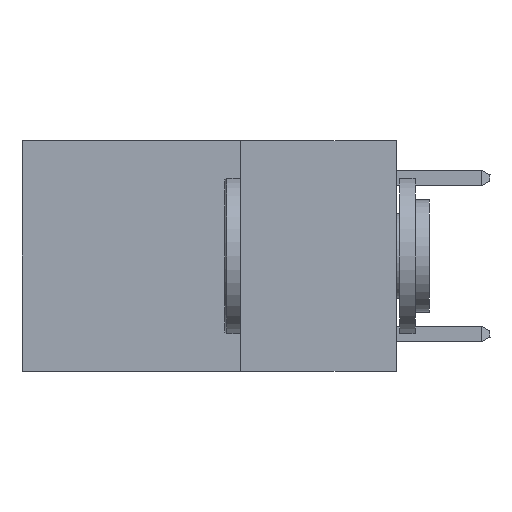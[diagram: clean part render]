
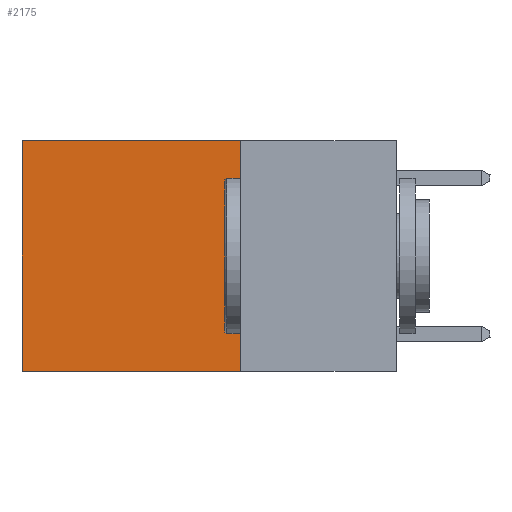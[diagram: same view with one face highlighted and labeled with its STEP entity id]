
A CAD part, left-side view. The second image highlights one B-rep face of the part: STEP entity #2175.
In plain terms, the highlighted planar face has unit normal (-1, 0, 0).
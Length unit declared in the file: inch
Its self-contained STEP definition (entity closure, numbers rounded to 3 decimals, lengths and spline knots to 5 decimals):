
#530 = CARTESIAN_POINT ( 'NONE',  ( 0.2625, 0.25, 0. ) ) ;
#537 = CARTESIAN_POINT ( 'NONE',  ( 0.2625, 0.6, -0.37 ) ) ;
#860 = VERTEX_POINT ( 'NONE', #9631 ) ;
#2175 = ADVANCED_FACE ( 'NONE', ( #6947 ), #11104, .F. ) ;
#2931 = DIRECTION ( 'NONE',  ( 0., 1., 0. ) ) ;
#3820 = ORIENTED_EDGE ( 'NONE', *, *, #22579, .F. ) ;
#5624 = VERTEX_POINT ( 'NONE', #16555 ) ;
#6626 = AXIS2_PLACEMENT_3D ( 'NONE', #17015, #23291, #23563 ) ;
#6947 = FACE_OUTER_BOUND ( 'NONE', #21028, .T. ) ;
#7235 = CARTESIAN_POINT ( 'NONE',  ( 0.2625, 0.25, -0.37 ) ) ;
#9631 = CARTESIAN_POINT ( 'NONE',  ( 0.2625, 0.25, -0.37 ) ) ;
#10124 = ORIENTED_EDGE ( 'NONE', *, *, #22635, .F. ) ;
#10319 = LINE ( 'NONE', #18487, #22851 ) ;
#11104 = PLANE ( 'NONE',  #6626 ) ;
#12025 = EDGE_CURVE ( 'NONE', #23098, #22059, #10319, .T. ) ;
#12121 = VECTOR ( 'NONE', #2931, 39.37008 ) ;
#14465 = DIRECTION ( 'NONE',  ( 0., 0., -1. ) ) ;
#14521 = ORIENTED_EDGE ( 'NONE', *, *, #20691, .T. ) ;
#15416 = CARTESIAN_POINT ( 'NONE',  ( 0.2625, 0.25, 0. ) ) ;
#16464 = ORIENTED_EDGE ( 'NONE', *, *, #12025, .T. ) ;
#16555 = CARTESIAN_POINT ( 'NONE',  ( 0.2625, 0.25, 0. ) ) ;
#17015 = CARTESIAN_POINT ( 'NONE',  ( 0.2625, 0.25, 0. ) ) ;
#17694 = VECTOR ( 'NONE', #21559, 39.37008 ) ;
#18487 = CARTESIAN_POINT ( 'NONE',  ( 0.2625, 0.6, 0. ) ) ;
#18525 = VECTOR ( 'NONE', #22793, 39.37008 ) ;
#19422 = LINE ( 'NONE', #15416, #17694 ) ;
#20095 = CARTESIAN_POINT ( 'NONE',  ( 0.2625, 0.6, 0. ) ) ;
#20648 = LINE ( 'NONE', #530, #18525 ) ;
#20691 = EDGE_CURVE ( 'NONE', #5624, #23098, #20648, .T. ) ;
#21028 = EDGE_LOOP ( 'NONE', ( #16464, #3820, #10124, #14521 ) ) ;
#21295 = LINE ( 'NONE', #7235, #12121 ) ;
#21559 = DIRECTION ( 'NONE',  ( 0., 0., -1. ) ) ;
#22059 = VERTEX_POINT ( 'NONE', #537 ) ;
#22579 = EDGE_CURVE ( 'NONE', #860, #22059, #21295, .T. ) ;
#22635 = EDGE_CURVE ( 'NONE', #5624, #860, #19422, .T. ) ;
#22793 = DIRECTION ( 'NONE',  ( 0., 1., 0. ) ) ;
#22851 = VECTOR ( 'NONE', #14465, 39.37008 ) ;
#23098 = VERTEX_POINT ( 'NONE', #20095 ) ;
#23291 = DIRECTION ( 'NONE',  ( 1., 0., 0. ) ) ;
#23563 = DIRECTION ( 'NONE',  ( 0., 0., -1. ) ) ;
